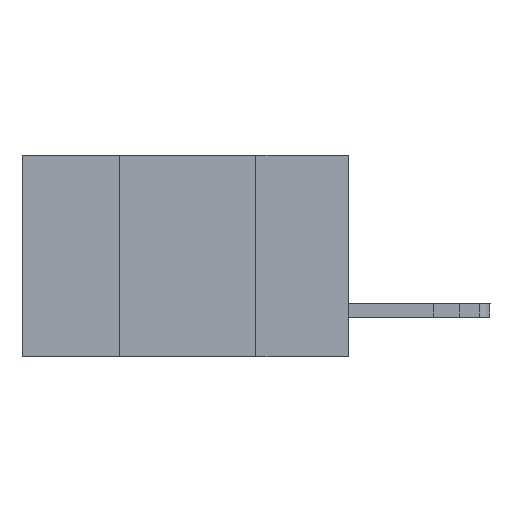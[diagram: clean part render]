
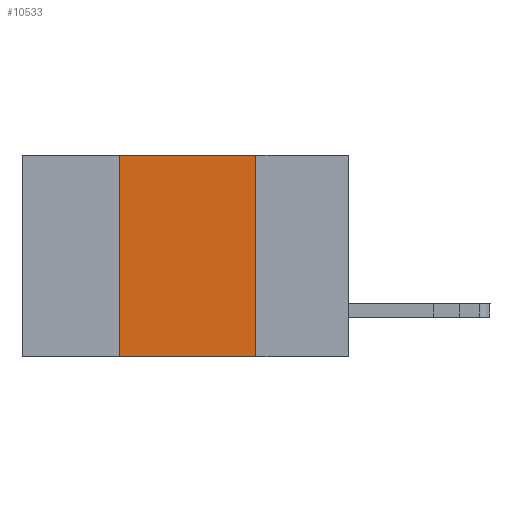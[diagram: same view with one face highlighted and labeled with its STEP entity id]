
A CAD part, left-side view. The second image highlights one B-rep face of the part: STEP entity #10533.
In plain terms, the highlighted planar face has unit normal (-1, 0, 0).
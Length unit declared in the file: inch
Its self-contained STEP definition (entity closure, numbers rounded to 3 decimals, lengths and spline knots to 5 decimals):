
#294 = EDGE_CURVE ( 'NONE', #2307, #11062, #11297, .T. ) ;
#1008 = ORIENTED_EDGE ( 'NONE', *, *, #294, .F. ) ;
#1032 = CARTESIAN_POINT ( 'NONE',  ( 0., 0.42, -0.37 ) ) ;
#1261 = VECTOR ( 'NONE', #6410, 39.37008 ) ;
#1340 = VECTOR ( 'NONE', #9864, 39.37008 ) ;
#1617 = CARTESIAN_POINT ( 'NONE',  ( 0., 0.42, 0. ) ) ;
#1659 = CARTESIAN_POINT ( 'NONE',  ( 0., 0.17, 0. ) ) ;
#1838 = PLANE ( 'NONE',  #8756 ) ;
#2307 = VERTEX_POINT ( 'NONE', #1032 ) ;
#2936 = DIRECTION ( 'NONE',  ( 1., 0., 0. ) ) ;
#3329 = ORIENTED_EDGE ( 'NONE', *, *, #10870, .T. ) ;
#3620 = FACE_OUTER_BOUND ( 'NONE', #4108, .T. ) ;
#3810 = VERTEX_POINT ( 'NONE', #8236 ) ;
#4108 = EDGE_LOOP ( 'NONE', ( #4530, #7896, #1008, #3329 ) ) ;
#4148 = LINE ( 'NONE', #1659, #1261 ) ;
#4530 = ORIENTED_EDGE ( 'NONE', *, *, #8131, .F. ) ;
#4647 = DIRECTION ( 'NONE',  ( 0., -1., 0. ) ) ;
#5517 = EDGE_CURVE ( 'NONE', #11062, #3810, #10810, .T. ) ;
#5657 = CARTESIAN_POINT ( 'NONE',  ( 0., 0.6, 0. ) ) ;
#5724 = CARTESIAN_POINT ( 'NONE',  ( 0., 0.6, 0. ) ) ;
#6143 = CARTESIAN_POINT ( 'NONE',  ( 0., 0.6, -0.37 ) ) ;
#6272 = LINE ( 'NONE', #6143, #1340 ) ;
#6398 = VERTEX_POINT ( 'NONE', #10673 ) ;
#6410 = DIRECTION ( 'NONE',  ( 0., 0., -1. ) ) ;
#7307 = VECTOR ( 'NONE', #12053, 39.37008 ) ;
#7408 = CARTESIAN_POINT ( 'NONE',  ( 0., 0.42, 0. ) ) ;
#7419 = VECTOR ( 'NONE', #4647, 39.37008 ) ;
#7896 = ORIENTED_EDGE ( 'NONE', *, *, #5517, .F. ) ;
#8131 = EDGE_CURVE ( 'NONE', #3810, #6398, #4148, .T. ) ;
#8236 = CARTESIAN_POINT ( 'NONE',  ( 0., 0.17, 0. ) ) ;
#8756 = AXIS2_PLACEMENT_3D ( 'NONE', #5724, #2936, #9492 ) ;
#9492 = DIRECTION ( 'NONE',  ( 0., 0., -1. ) ) ;
#9864 = DIRECTION ( 'NONE',  ( 0., -1., 0. ) ) ;
#10533 = ADVANCED_FACE ( 'NONE', ( #3620 ), #1838, .F. ) ;
#10673 = CARTESIAN_POINT ( 'NONE',  ( 0., 0.17, -0.37 ) ) ;
#10810 = LINE ( 'NONE', #5657, #7419 ) ;
#10870 = EDGE_CURVE ( 'NONE', #2307, #6398, #6272, .T. ) ;
#11062 = VERTEX_POINT ( 'NONE', #1617 ) ;
#11297 = LINE ( 'NONE', #7408, #7307 ) ;
#12053 = DIRECTION ( 'NONE',  ( 0., 0., 1. ) ) ;
